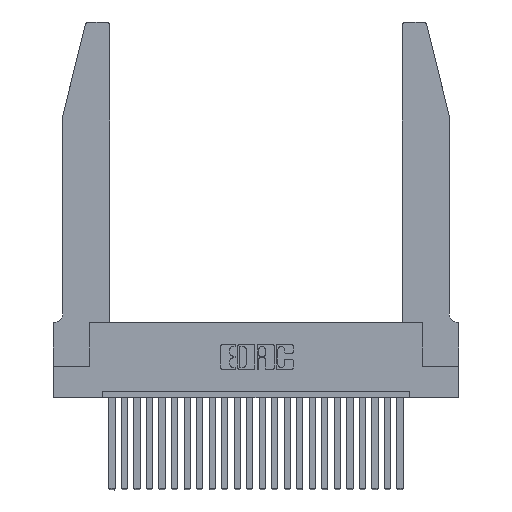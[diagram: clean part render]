
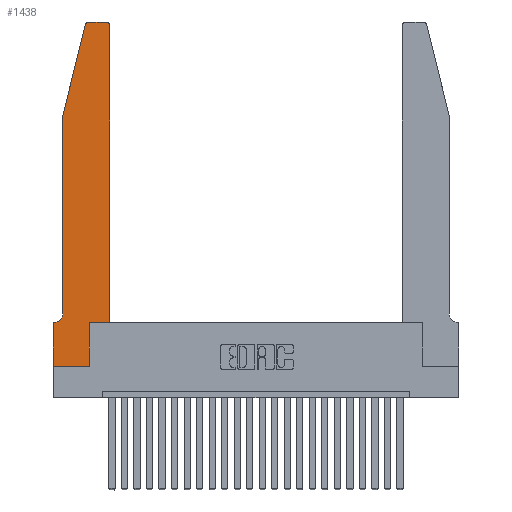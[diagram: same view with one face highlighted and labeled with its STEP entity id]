
A CAD part, top view. The second image highlights one B-rep face of the part: STEP entity #1438.
In plain terms, the highlighted planar face has unit normal (0, 0, 1).
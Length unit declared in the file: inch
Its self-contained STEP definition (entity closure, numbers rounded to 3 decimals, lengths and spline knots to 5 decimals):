
#445 = EDGE_LOOP ( 'NONE', ( #21299, #15283, #13120, #17542, #4281, #13445, #15862, #6560, #1104, #4260, #10022, #19419 ) ) ;
#1104 = ORIENTED_EDGE ( 'NONE', *, *, #13090, .T. ) ;
#1348 = VERTEX_POINT ( 'NONE', #2542 ) ;
#1438 = ADVANCED_FACE ( 'NONE', ( #2029 ), #6784, .T. ) ;
#1889 = DIRECTION ( 'NONE',  ( 0., 1., 0. ) ) ;
#2029 = FACE_OUTER_BOUND ( 'NONE', #445, .T. ) ;
#2058 = VERTEX_POINT ( 'NONE', #12470 ) ;
#2130 = CIRCLE ( 'NONE', #10672, 0.03 ) ;
#2301 = CARTESIAN_POINT ( 'NONE',  ( 0., 0., 0.37 ) ) ;
#2339 = VECTOR ( 'NONE', #18813, 39.37008 ) ;
#2379 = DIRECTION ( 'NONE',  ( 1., 0., 0. ) ) ;
#2542 = CARTESIAN_POINT ( 'NONE',  ( 0., 0.35, 0.37 ) ) ;
#2554 = EDGE_CURVE ( 'NONE', #14202, #12306, #7482, .T. ) ;
#2785 = CARTESIAN_POINT ( 'NONE',  ( 0.284, 2.75, 0.37 ) ) ;
#3017 = VECTOR ( 'NONE', #20248, 39.37008 ) ;
#3911 = LINE ( 'NONE', #2301, #6336 ) ;
#3932 = LINE ( 'NONE', #13160, #23830 ) ;
#4260 = ORIENTED_EDGE ( 'NONE', *, *, #7943, .T. ) ;
#4281 = ORIENTED_EDGE ( 'NONE', *, *, #2554, .T. ) ;
#4369 = DIRECTION ( 'NONE',  ( 0., -1., 0. ) ) ;
#4453 = VECTOR ( 'NONE', #23007, 39.37008 ) ;
#5321 = VERTEX_POINT ( 'NONE', #20637 ) ;
#5653 = CARTESIAN_POINT ( 'NONE',  ( 0.4505, 0.35, 0.37 ) ) ;
#5745 = EDGE_CURVE ( 'NONE', #17821, #2058, #2130, .T. ) ;
#5894 = DIRECTION ( 'NONE',  ( 0., 0., 1. ) ) ;
#6186 = VECTOR ( 'NONE', #14574, 39.37008 ) ;
#6336 = VECTOR ( 'NONE', #2379, 39.37008 ) ;
#6558 = AXIS2_PLACEMENT_3D ( 'NONE', #6872, #20261, #14594 ) ;
#6560 = ORIENTED_EDGE ( 'NONE', *, *, #13335, .T. ) ;
#6643 = CARTESIAN_POINT ( 'NONE',  ( 0.2865, 0.35, 0.37 ) ) ;
#6784 = PLANE ( 'NONE',  #6558 ) ;
#6872 = CARTESIAN_POINT ( 'NONE',  ( 0., 0.35, 0.37 ) ) ;
#6907 = DIRECTION ( 'NONE',  ( -1., 0., 0. ) ) ;
#7215 = CARTESIAN_POINT ( 'NONE',  ( 0.4205, 2.72, 0.37 ) ) ;
#7293 = EDGE_CURVE ( 'NONE', #24707, #17821, #16574, .T. ) ;
#7482 = CIRCLE ( 'NONE', #7894, 0.07 ) ;
#7500 = VECTOR ( 'NONE', #4369, 39.37008 ) ;
#7710 = CARTESIAN_POINT ( 'NONE',  ( 0.4505, 2.72, 0.37 ) ) ;
#7721 = EDGE_CURVE ( 'NONE', #23561, #14945, #12615, .T. ) ;
#7852 = CARTESIAN_POINT ( 'NONE',  ( 0.25487, 2.72718, 0.37 ) ) ;
#7873 = EDGE_CURVE ( 'NONE', #14945, #14202, #16842, .T. ) ;
#7894 = AXIS2_PLACEMENT_3D ( 'NONE', #16328, #20293, #6907 ) ;
#7943 = EDGE_CURVE ( 'NONE', #12094, #24707, #21990, .T. ) ;
#8036 = EDGE_CURVE ( 'NONE', #1348, #8057, #10512, .T. ) ;
#8057 = VERTEX_POINT ( 'NONE', #20480 ) ;
#8255 = CARTESIAN_POINT ( 'NONE',  ( 0.284, 2.72, 0.37 ) ) ;
#9775 = DIRECTION ( 'NONE',  ( 1., 0., 0. ) ) ;
#9997 = DIRECTION ( 'NONE',  ( 0., -1., 0. ) ) ;
#10022 = ORIENTED_EDGE ( 'NONE', *, *, #7293, .T. ) ;
#10512 = LINE ( 'NONE', #18537, #7500 ) ;
#10672 = AXIS2_PLACEMENT_3D ( 'NONE', #7215, #20678, #22640 ) ;
#10823 = CARTESIAN_POINT ( 'NONE',  ( 0.2605, 2.75, 0.37 ) ) ;
#11821 = CARTESIAN_POINT ( 'NONE',  ( 0.0755, 2., 0.37 ) ) ;
#12094 = VERTEX_POINT ( 'NONE', #6643 ) ;
#12306 = VERTEX_POINT ( 'NONE', #18309 ) ;
#12470 = CARTESIAN_POINT ( 'NONE',  ( 0.4205, 2.75, 0.37 ) ) ;
#12615 = LINE ( 'NONE', #22787, #2339 ) ;
#13090 = EDGE_CURVE ( 'NONE', #5321, #12094, #3932, .T. ) ;
#13120 = ORIENTED_EDGE ( 'NONE', *, *, #7721, .T. ) ;
#13121 = LINE ( 'NONE', #16531, #6186 ) ;
#13160 = CARTESIAN_POINT ( 'NONE',  ( 0.2865, 0.35, 0.37 ) ) ;
#13335 = EDGE_CURVE ( 'NONE', #8057, #5321, #3911, .T. ) ;
#13445 = ORIENTED_EDGE ( 'NONE', *, *, #13863, .T. ) ;
#13795 = VECTOR ( 'NONE', #9997, 39.37008 ) ;
#13863 = EDGE_CURVE ( 'NONE', #12306, #1348, #13121, .T. ) ;
#14202 = VERTEX_POINT ( 'NONE', #15655 ) ;
#14574 = DIRECTION ( 'NONE',  ( -1., 0., 0. ) ) ;
#14594 = DIRECTION ( 'NONE',  ( 1., 0., 0. ) ) ;
#14945 = VERTEX_POINT ( 'NONE', #11821 ) ;
#15237 = CARTESIAN_POINT ( 'NONE',  ( 0.4505, 0.35, 0.37 ) ) ;
#15283 = ORIENTED_EDGE ( 'NONE', *, *, #19193, .T. ) ;
#15655 = CARTESIAN_POINT ( 'NONE',  ( 0.0755, 0.42, 0.37 ) ) ;
#15862 = ORIENTED_EDGE ( 'NONE', *, *, #8036, .T. ) ;
#16328 = CARTESIAN_POINT ( 'NONE',  ( 0.0055, 0.42, 0.37 ) ) ;
#16531 = CARTESIAN_POINT ( 'NONE',  ( 0.0755, 0.35, 0.37 ) ) ;
#16574 = LINE ( 'NONE', #15237, #20175 ) ;
#16842 = LINE ( 'NONE', #17486, #13795 ) ;
#17486 = CARTESIAN_POINT ( 'NONE',  ( 0.0755, 2., 0.37 ) ) ;
#17542 = ORIENTED_EDGE ( 'NONE', *, *, #7873, .T. ) ;
#17821 = VERTEX_POINT ( 'NONE', #7710 ) ;
#18309 = CARTESIAN_POINT ( 'NONE',  ( 0.0055, 0.35, 0.37 ) ) ;
#18537 = CARTESIAN_POINT ( 'NONE',  ( 0., 0., 0.37 ) ) ;
#18813 = DIRECTION ( 'NONE',  ( -0.239, -0.971, 0. ) ) ;
#18991 = DIRECTION ( 'NONE',  ( 0., 1., 0. ) ) ;
#19193 = EDGE_CURVE ( 'NONE', #20416, #23561, #20975, .T. ) ;
#19419 = ORIENTED_EDGE ( 'NONE', *, *, #5745, .T. ) ;
#19680 = AXIS2_PLACEMENT_3D ( 'NONE', #8255, #5894, #9775 ) ;
#20175 = VECTOR ( 'NONE', #1889, 39.37008 ) ;
#20248 = DIRECTION ( 'NONE',  ( -1., 0., 0. ) ) ;
#20261 = DIRECTION ( 'NONE',  ( 0., 0., 1. ) ) ;
#20293 = DIRECTION ( 'NONE',  ( 0., 0., -1. ) ) ;
#20416 = VERTEX_POINT ( 'NONE', #2785 ) ;
#20480 = CARTESIAN_POINT ( 'NONE',  ( 0., 0., 0.37 ) ) ;
#20637 = CARTESIAN_POINT ( 'NONE',  ( 0.2865, 0., 0.37 ) ) ;
#20678 = DIRECTION ( 'NONE',  ( 0., 0., 1. ) ) ;
#20975 = CIRCLE ( 'NONE', #19680, 0.03 ) ;
#21299 = ORIENTED_EDGE ( 'NONE', *, *, #21479, .T. ) ;
#21479 = EDGE_CURVE ( 'NONE', #2058, #20416, #22647, .T. ) ;
#21990 = LINE ( 'NONE', #5653, #4453 ) ;
#22640 = DIRECTION ( 'NONE',  ( 1., 0., 0. ) ) ;
#22647 = LINE ( 'NONE', #10823, #3017 ) ;
#22787 = CARTESIAN_POINT ( 'NONE',  ( 0.0755, 2., 0.37 ) ) ;
#23007 = DIRECTION ( 'NONE',  ( 1., 0., 0. ) ) ;
#23561 = VERTEX_POINT ( 'NONE', #7852 ) ;
#23830 = VECTOR ( 'NONE', #18991, 39.37008 ) ;
#24399 = CARTESIAN_POINT ( 'NONE',  ( 0.4505, 0.35, 0.37 ) ) ;
#24707 = VERTEX_POINT ( 'NONE', #24399 ) ;
